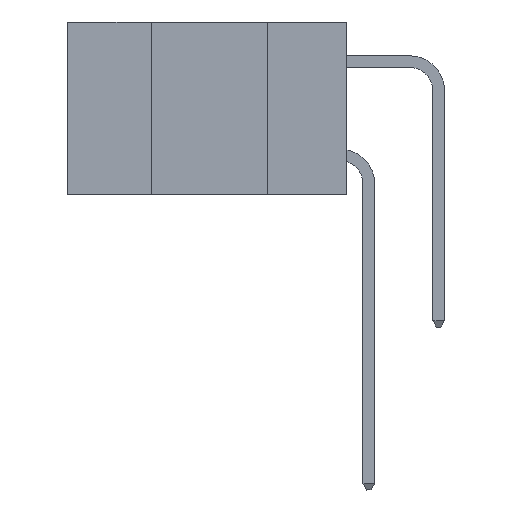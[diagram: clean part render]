
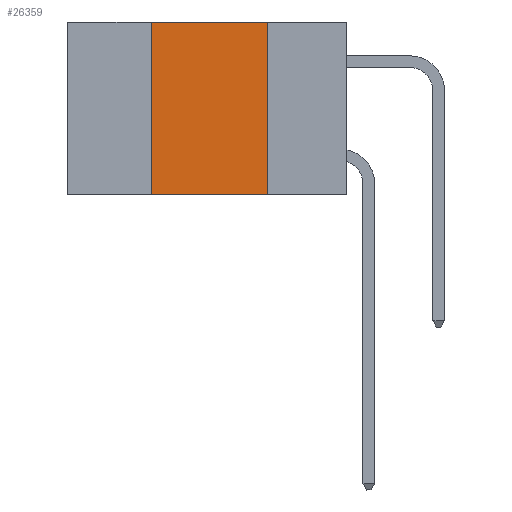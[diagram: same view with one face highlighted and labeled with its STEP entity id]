
A CAD part, left-side view. The second image highlights one B-rep face of the part: STEP entity #26359.
In plain terms, the highlighted planar face has unit normal (-1, 0, 0).
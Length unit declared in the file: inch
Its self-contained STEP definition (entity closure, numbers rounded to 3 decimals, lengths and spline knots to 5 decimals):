
#351 = LINE ( 'NONE', #8291, #28303 ) ;
#801 = ORIENTED_EDGE ( 'NONE', *, *, #1161, .T. ) ;
#1053 = DIRECTION ( 'NONE',  ( 0., 0., -1. ) ) ;
#1161 = EDGE_CURVE ( 'NONE', #9741, #9240, #351, .T. ) ;
#1235 = DIRECTION ( 'NONE',  ( 1., 0., 0. ) ) ;
#2025 = DIRECTION ( 'NONE',  ( 0., -1., 0. ) ) ;
#3426 = EDGE_CURVE ( 'NONE', #9741, #28080, #25007, .T. ) ;
#5161 = LINE ( 'NONE', #12017, #28203 ) ;
#6277 = CARTESIAN_POINT ( 'NONE',  ( 0., 0.17, -0.37 ) ) ;
#7734 = LINE ( 'NONE', #13756, #13335 ) ;
#8108 = CARTESIAN_POINT ( 'NONE',  ( 0., 0.42, -0.37 ) ) ;
#8291 = CARTESIAN_POINT ( 'NONE',  ( 0., 0.6, -0.37 ) ) ;
#9172 = EDGE_LOOP ( 'NONE', ( #22611, #21391, #25920, #801 ) ) ;
#9240 = VERTEX_POINT ( 'NONE', #6277 ) ;
#9741 = VERTEX_POINT ( 'NONE', #8108 ) ;
#12017 = CARTESIAN_POINT ( 'NONE',  ( 0., 0.17, 0. ) ) ;
#12061 = EDGE_CURVE ( 'NONE', #28080, #14341, #7734, .T. ) ;
#13335 = VECTOR ( 'NONE', #15738, 39.37008 ) ;
#13756 = CARTESIAN_POINT ( 'NONE',  ( 0., 0.6, 0. ) ) ;
#14341 = VERTEX_POINT ( 'NONE', #18939 ) ;
#15738 = DIRECTION ( 'NONE',  ( 0., -1., 0. ) ) ;
#16802 = CARTESIAN_POINT ( 'NONE',  ( 0., 0.6, 0. ) ) ;
#17771 = CARTESIAN_POINT ( 'NONE',  ( 0., 0.42, 0. ) ) ;
#18939 = CARTESIAN_POINT ( 'NONE',  ( 0., 0.17, 0. ) ) ;
#19107 = VECTOR ( 'NONE', #22264, 39.37008 ) ;
#21178 = DIRECTION ( 'NONE',  ( 0., 0., -1. ) ) ;
#21391 = ORIENTED_EDGE ( 'NONE', *, *, #12061, .F. ) ;
#21867 = FACE_OUTER_BOUND ( 'NONE', #9172, .T. ) ;
#22264 = DIRECTION ( 'NONE',  ( 0., 0., 1. ) ) ;
#22611 = ORIENTED_EDGE ( 'NONE', *, *, #24975, .F. ) ;
#24975 = EDGE_CURVE ( 'NONE', #14341, #9240, #5161, .T. ) ;
#25007 = LINE ( 'NONE', #17771, #19107 ) ;
#25386 = CARTESIAN_POINT ( 'NONE',  ( 0., 0.42, 0. ) ) ;
#25920 = ORIENTED_EDGE ( 'NONE', *, *, #3426, .F. ) ;
#26359 = ADVANCED_FACE ( 'NONE', ( #21867 ), #27896, .F. ) ;
#26827 = AXIS2_PLACEMENT_3D ( 'NONE', #16802, #1235, #21178 ) ;
#27896 = PLANE ( 'NONE',  #26827 ) ;
#28080 = VERTEX_POINT ( 'NONE', #25386 ) ;
#28203 = VECTOR ( 'NONE', #1053, 39.37008 ) ;
#28303 = VECTOR ( 'NONE', #2025, 39.37008 ) ;
